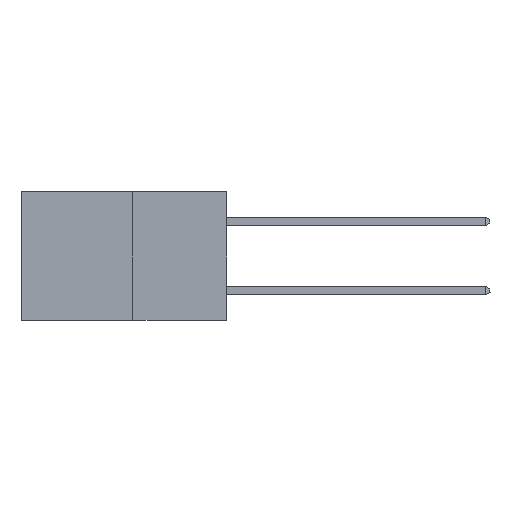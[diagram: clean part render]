
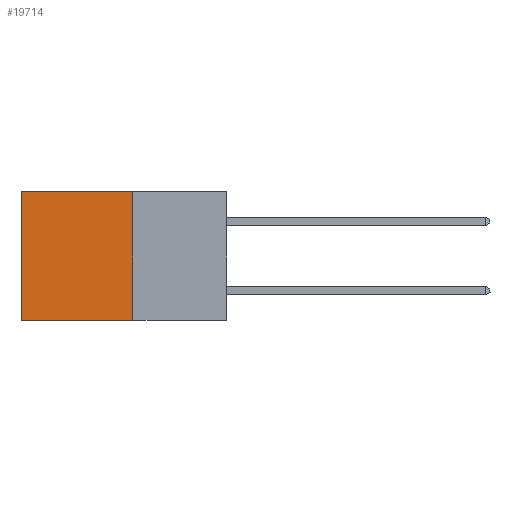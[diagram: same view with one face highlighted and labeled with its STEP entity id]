
A CAD part, left-side view. The second image highlights one B-rep face of the part: STEP entity #19714.
In plain terms, the highlighted planar face has unit normal (-1, 0, 0).
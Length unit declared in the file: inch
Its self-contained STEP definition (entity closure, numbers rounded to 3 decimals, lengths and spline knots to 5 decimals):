
#205 = DIRECTION ( 'NONE',  ( 0., 0., -1. ) ) ;
#1017 = LINE ( 'NONE', #7371, #14411 ) ;
#1230 = DIRECTION ( 'NONE',  ( 0., 0., -1. ) ) ;
#1326 = CARTESIAN_POINT ( 'NONE',  ( 0.277, 0.27, 0. ) ) ;
#1506 = EDGE_LOOP ( 'NONE', ( #17977, #15184, #11906, #17685 ) ) ;
#2199 = CARTESIAN_POINT ( 'NONE',  ( 0.277, 0.27, -0.37 ) ) ;
#2370 = VECTOR ( 'NONE', #17840, 39.37008 ) ;
#3209 = VERTEX_POINT ( 'NONE', #1326 ) ;
#3881 = EDGE_CURVE ( 'NONE', #20435, #15865, #5333, .T. ) ;
#4044 = DIRECTION ( 'NONE',  ( 0., 1., 0. ) ) ;
#4774 = VECTOR ( 'NONE', #1230, 39.37008 ) ;
#5333 = LINE ( 'NONE', #18599, #4774 ) ;
#5459 = CARTESIAN_POINT ( 'NONE',  ( 0.277, 0.59, 0. ) ) ;
#5493 = VERTEX_POINT ( 'NONE', #21069 ) ;
#6375 = CARTESIAN_POINT ( 'NONE',  ( 0.277, 0.59, -0.37 ) ) ;
#7260 = EDGE_CURVE ( 'NONE', #3209, #5493, #7593, .T. ) ;
#7371 = CARTESIAN_POINT ( 'NONE',  ( 0.277, 0.27, -0.37 ) ) ;
#7593 = LINE ( 'NONE', #2199, #2370 ) ;
#10691 = DIRECTION ( 'NONE',  ( 1., 0., 0. ) ) ;
#11906 = ORIENTED_EDGE ( 'NONE', *, *, #7260, .F. ) ;
#13588 = EDGE_CURVE ( 'NONE', #5493, #15865, #1017, .T. ) ;
#14109 = PLANE ( 'NONE',  #17889 ) ;
#14411 = VECTOR ( 'NONE', #16002, 39.37008 ) ;
#14564 = LINE ( 'NONE', #19678, #18628 ) ;
#15184 = ORIENTED_EDGE ( 'NONE', *, *, #13588, .F. ) ;
#15865 = VERTEX_POINT ( 'NONE', #6375 ) ;
#16002 = DIRECTION ( 'NONE',  ( 0., 1., 0. ) ) ;
#17685 = ORIENTED_EDGE ( 'NONE', *, *, #20520, .T. ) ;
#17840 = DIRECTION ( 'NONE',  ( 0., 0., -1. ) ) ;
#17889 = AXIS2_PLACEMENT_3D ( 'NONE', #21034, #10691, #205 ) ;
#17977 = ORIENTED_EDGE ( 'NONE', *, *, #3881, .T. ) ;
#18599 = CARTESIAN_POINT ( 'NONE',  ( 0.277, 0.59, -0.37 ) ) ;
#18628 = VECTOR ( 'NONE', #4044, 39.37008 ) ;
#19678 = CARTESIAN_POINT ( 'NONE',  ( 0.277, 0.27, 0. ) ) ;
#19714 = ADVANCED_FACE ( 'NONE', ( #21583 ), #14109, .F. ) ;
#20435 = VERTEX_POINT ( 'NONE', #5459 ) ;
#20520 = EDGE_CURVE ( 'NONE', #3209, #20435, #14564, .T. ) ;
#21034 = CARTESIAN_POINT ( 'NONE',  ( 0.277, 0.27, -0.37 ) ) ;
#21069 = CARTESIAN_POINT ( 'NONE',  ( 0.277, 0.27, -0.37 ) ) ;
#21583 = FACE_OUTER_BOUND ( 'NONE', #1506, .T. ) ;
